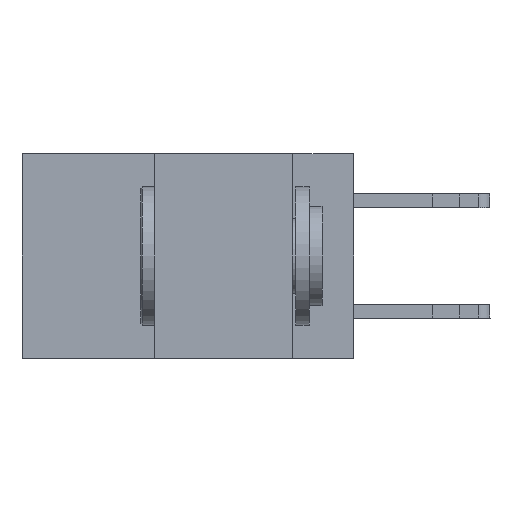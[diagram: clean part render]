
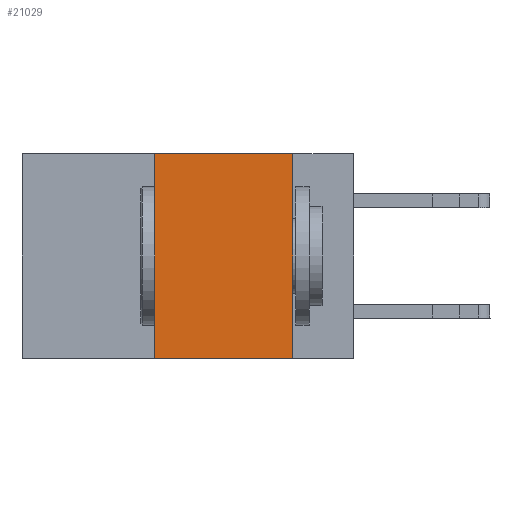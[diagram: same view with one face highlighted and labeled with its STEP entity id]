
A CAD part, left-side view. The second image highlights one B-rep face of the part: STEP entity #21029.
In plain terms, the highlighted planar face has unit normal (-1, 0, 0).
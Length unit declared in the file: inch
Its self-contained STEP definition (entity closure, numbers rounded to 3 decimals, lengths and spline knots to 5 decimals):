
#612 = LINE ( 'NONE', #17256, #18186 ) ;
#683 = EDGE_CURVE ( 'NONE', #7994, #24662, #16734, .T. ) ;
#879 = VERTEX_POINT ( 'NONE', #15607 ) ;
#1354 = CARTESIAN_POINT ( 'NONE',  ( 0., 0.36, 0. ) ) ;
#2907 = VERTEX_POINT ( 'NONE', #3982 ) ;
#3982 = CARTESIAN_POINT ( 'NONE',  ( 0., 0.36, 0. ) ) ;
#4364 = LINE ( 'NONE', #23342, #21720 ) ;
#4764 = ORIENTED_EDGE ( 'NONE', *, *, #20000, .F. ) ;
#5841 = ORIENTED_EDGE ( 'NONE', *, *, #26824, .F. ) ;
#7050 = EDGE_CURVE ( 'NONE', #2907, #879, #4364, .T. ) ;
#7672 = DIRECTION ( 'NONE',  ( 0., 0., -1. ) ) ;
#7994 = VERTEX_POINT ( 'NONE', #26509 ) ;
#9503 = DIRECTION ( 'NONE',  ( 0., 0., 1. ) ) ;
#9882 = FACE_OUTER_BOUND ( 'NONE', #20968, .T. ) ;
#11931 = LINE ( 'NONE', #1354, #23408 ) ;
#13872 = ORIENTED_EDGE ( 'NONE', *, *, #683, .T. ) ;
#14256 = DIRECTION ( 'NONE',  ( 0., -1., 0. ) ) ;
#14520 = CARTESIAN_POINT ( 'NONE',  ( 0., 0.6, -0.37 ) ) ;
#15343 = DIRECTION ( 'NONE',  ( 0., -1., 0. ) ) ;
#15607 = CARTESIAN_POINT ( 'NONE',  ( 0., 0.11, 0. ) ) ;
#15637 = CARTESIAN_POINT ( 'NONE',  ( 0., 0.6, 0. ) ) ;
#16734 = LINE ( 'NONE', #14520, #17007 ) ;
#17007 = VECTOR ( 'NONE', #14256, 39.37008 ) ;
#17256 = CARTESIAN_POINT ( 'NONE',  ( 0., 0.11, 0. ) ) ;
#18186 = VECTOR ( 'NONE', #25660, 39.37008 ) ;
#20000 = EDGE_CURVE ( 'NONE', #879, #24662, #612, .T. ) ;
#20968 = EDGE_LOOP ( 'NONE', ( #4764, #26886, #5841, #13872 ) ) ;
#21029 = ADVANCED_FACE ( 'NONE', ( #9882 ), #24323, .F. ) ;
#21720 = VECTOR ( 'NONE', #15343, 39.37008 ) ;
#22627 = AXIS2_PLACEMENT_3D ( 'NONE', #15637, #24467, #7672 ) ;
#23342 = CARTESIAN_POINT ( 'NONE',  ( 0., 0.6, 0. ) ) ;
#23408 = VECTOR ( 'NONE', #9503, 39.37008 ) ;
#24323 = PLANE ( 'NONE',  #22627 ) ;
#24467 = DIRECTION ( 'NONE',  ( 1., 0., 0. ) ) ;
#24662 = VERTEX_POINT ( 'NONE', #25479 ) ;
#25479 = CARTESIAN_POINT ( 'NONE',  ( 0., 0.11, -0.37 ) ) ;
#25660 = DIRECTION ( 'NONE',  ( 0., 0., -1. ) ) ;
#26509 = CARTESIAN_POINT ( 'NONE',  ( 0., 0.36, -0.37 ) ) ;
#26824 = EDGE_CURVE ( 'NONE', #7994, #2907, #11931, .T. ) ;
#26886 = ORIENTED_EDGE ( 'NONE', *, *, #7050, .F. ) ;
